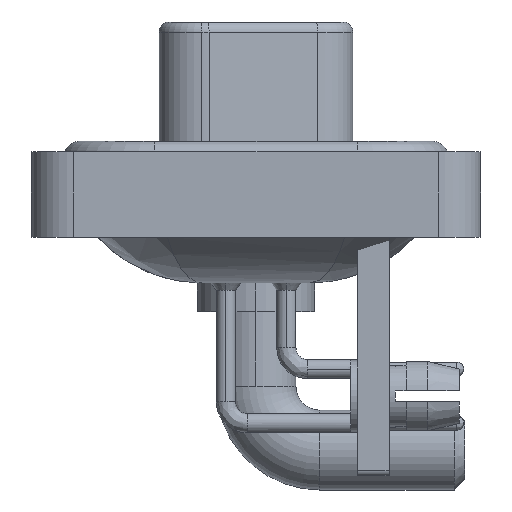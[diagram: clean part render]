
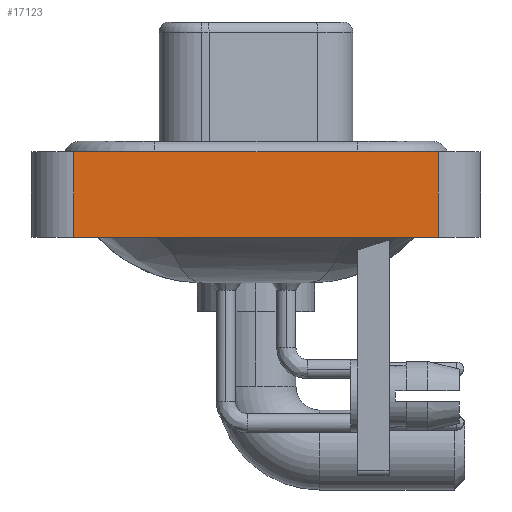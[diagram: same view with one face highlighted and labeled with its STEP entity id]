
A CAD part, left-side view. The second image highlights one B-rep face of the part: STEP entity #17123.
In plain terms, the highlighted planar face has unit normal (-1, 0, 0).
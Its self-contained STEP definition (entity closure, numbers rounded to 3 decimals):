
#958 = CARTESIAN_POINT ( 'NONE',  ( -7.25, -8.55, -3.6 ) ) ;
#1699 = CARTESIAN_POINT ( 'NONE',  ( -7.25, -8.55, 0.4 ) ) ;
#1927 = CARTESIAN_POINT ( 'NONE',  ( -7.25, 8.55, -3.6 ) ) ;
#2605 = EDGE_LOOP ( 'NONE', ( #12955, #19155, #13887, #11405 ) ) ;
#3713 = CARTESIAN_POINT ( 'NONE',  ( -7.25, -8.55, 0.4 ) ) ;
#3968 = LINE ( 'NONE', #9745, #6904 ) ;
#5371 = VECTOR ( 'NONE', #9485, 1000. ) ;
#6904 = VECTOR ( 'NONE', #21739, 1000. ) ;
#7075 = VERTEX_POINT ( 'NONE', #15185 ) ;
#8111 = CARTESIAN_POINT ( 'NONE',  ( -7.25, -8.55, -3.6 ) ) ;
#8358 = LINE ( 'NONE', #8111, #17008 ) ;
#8909 = AXIS2_PLACEMENT_3D ( 'NONE', #958, #18201, #17950 ) ;
#9485 = DIRECTION ( 'NONE',  ( 0., 0., 1. ) ) ;
#9745 = CARTESIAN_POINT ( 'NONE',  ( -7.25, -8.55, -3.6 ) ) ;
#9795 = DIRECTION ( 'NONE',  ( 0., 0., 1. ) ) ;
#11299 = VERTEX_POINT ( 'NONE', #19080 ) ;
#11405 = ORIENTED_EDGE ( 'NONE', *, *, #20395, .T. ) ;
#12571 = PLANE ( 'NONE',  #8909 ) ;
#12955 = ORIENTED_EDGE ( 'NONE', *, *, #24299, .T. ) ;
#13694 = VECTOR ( 'NONE', #19418, 1000. ) ;
#13887 = ORIENTED_EDGE ( 'NONE', *, *, #19159, .F. ) ;
#14126 = FACE_OUTER_BOUND ( 'NONE', #2605, .T. ) ;
#14336 = EDGE_CURVE ( 'NONE', #16372, #14768, #17264, .T. ) ;
#14768 = VERTEX_POINT ( 'NONE', #1699 ) ;
#15185 = CARTESIAN_POINT ( 'NONE',  ( -7.25, 8.55, -3.6 ) ) ;
#15613 = LINE ( 'NONE', #1927, #5371 ) ;
#16372 = VERTEX_POINT ( 'NONE', #24165 ) ;
#17008 = VECTOR ( 'NONE', #9795, 1000. ) ;
#17123 = ADVANCED_FACE ( 'NONE', ( #14126 ), #12571, .T. ) ;
#17264 = LINE ( 'NONE', #3713, #13694 ) ;
#17950 = DIRECTION ( 'NONE',  ( 0., 0., 1. ) ) ;
#18201 = DIRECTION ( 'NONE',  ( -1., 0., 0. ) ) ;
#19080 = CARTESIAN_POINT ( 'NONE',  ( -7.25, -8.55, -3.6 ) ) ;
#19155 = ORIENTED_EDGE ( 'NONE', *, *, #14336, .F. ) ;
#19159 = EDGE_CURVE ( 'NONE', #7075, #16372, #15613, .T. ) ;
#19418 = DIRECTION ( 'NONE',  ( 0., -1., 0. ) ) ;
#20395 = EDGE_CURVE ( 'NONE', #7075, #11299, #3968, .T. ) ;
#21739 = DIRECTION ( 'NONE',  ( 0., -1., 0. ) ) ;
#24165 = CARTESIAN_POINT ( 'NONE',  ( -7.25, 8.55, 0.4 ) ) ;
#24299 = EDGE_CURVE ( 'NONE', #11299, #14768, #8358, .T. ) ;
